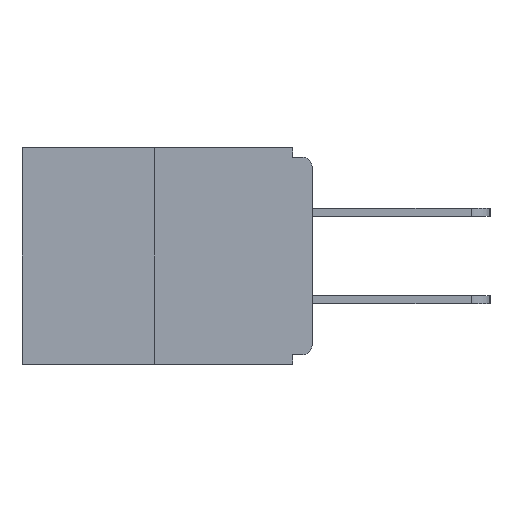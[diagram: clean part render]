
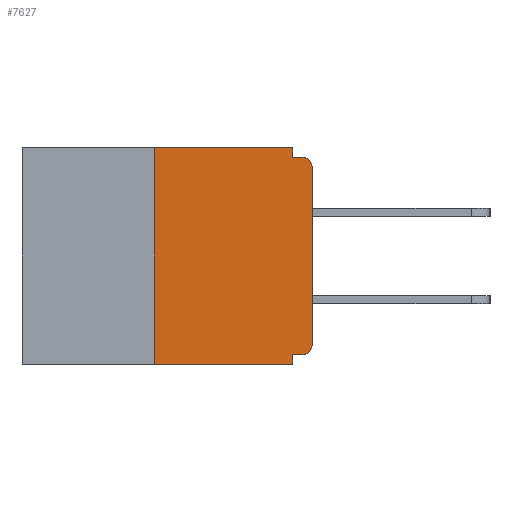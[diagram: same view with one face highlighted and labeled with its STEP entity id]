
A CAD part, left-side view. The second image highlights one B-rep face of the part: STEP entity #7627.
In plain terms, the highlighted planar face has unit normal (-1, 0, 0).
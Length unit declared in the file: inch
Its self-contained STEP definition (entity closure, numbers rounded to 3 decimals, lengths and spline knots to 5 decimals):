
#273 = ORIENTED_EDGE ( 'NONE', *, *, #18826, .F. ) ;
#470 = EDGE_LOOP ( 'NONE', ( #4976, #16208, #1547, #25998, #273, #16233, #20205, #10262, #1026, #14381 ) ) ;
#870 = VECTOR ( 'NONE', #19834, 39.37008 ) ;
#945 = DIRECTION ( 'NONE',  ( 1., 0., 0. ) ) ;
#1026 = ORIENTED_EDGE ( 'NONE', *, *, #16231, .F. ) ;
#1203 = DIRECTION ( 'NONE',  ( 0., 0., -1. ) ) ;
#1547 = ORIENTED_EDGE ( 'NONE', *, *, #17357, .T. ) ;
#2032 = VECTOR ( 'NONE', #5694, 39.37008 ) ;
#2045 = DIRECTION ( 'NONE',  ( 0., 0., 1. ) ) ;
#2410 = CARTESIAN_POINT ( 'NONE',  ( 0., 0.015, -0.313 ) ) ;
#3514 = DIRECTION ( 'NONE',  ( 0., -1., 0. ) ) ;
#3587 = LINE ( 'NONE', #8231, #18515 ) ;
#4628 = DIRECTION ( 'NONE',  ( -1., 0., 0. ) ) ;
#4914 = EDGE_CURVE ( 'NONE', #7676, #7644, #20408, .T. ) ;
#4976 = ORIENTED_EDGE ( 'NONE', *, *, #7115, .F. ) ;
#5045 = CARTESIAN_POINT ( 'NONE',  ( 0., 0.031, -0.015 ) ) ;
#5095 = EDGE_CURVE ( 'NONE', #22846, #19118, #3587, .T. ) ;
#5694 = DIRECTION ( 'NONE',  ( 0., -1., 0. ) ) ;
#6018 = CARTESIAN_POINT ( 'NONE',  ( 0., 0.031, 0. ) ) ;
#6121 = AXIS2_PLACEMENT_3D ( 'NONE', #2410, #4628, #24549 ) ;
#6451 = DIRECTION ( 'NONE',  ( -1., 0., 0. ) ) ;
#7105 = PLANE ( 'NONE',  #16457 ) ;
#7115 = EDGE_CURVE ( 'NONE', #15376, #7676, #24294, .T. ) ;
#7213 = CIRCLE ( 'NONE', #6121, 0.015 ) ;
#7627 = ADVANCED_FACE ( 'NONE', ( #17878 ), #7105, .F. ) ;
#7644 = VERTEX_POINT ( 'NONE', #5045 ) ;
#7676 = VERTEX_POINT ( 'NONE', #6018 ) ;
#7841 = CARTESIAN_POINT ( 'NONE',  ( 0., 0.46, 0. ) ) ;
#8231 = CARTESIAN_POINT ( 'NONE',  ( 0., 0., 0. ) ) ;
#8272 = CARTESIAN_POINT ( 'NONE',  ( 0., 0.015, -0.328 ) ) ;
#8774 = VERTEX_POINT ( 'NONE', #12982 ) ;
#8890 = LINE ( 'NONE', #25991, #870 ) ;
#8974 = CARTESIAN_POINT ( 'NONE',  ( 0., 0.015, -0.015 ) ) ;
#9414 = LINE ( 'NONE', #15908, #13529 ) ;
#9775 = DIRECTION ( 'NONE',  ( 0., 0., 1. ) ) ;
#10262 = ORIENTED_EDGE ( 'NONE', *, *, #13984, .T. ) ;
#11109 = CARTESIAN_POINT ( 'NONE',  ( 0., 0.46, 0. ) ) ;
#11891 = VERTEX_POINT ( 'NONE', #17225 ) ;
#12394 = AXIS2_PLACEMENT_3D ( 'NONE', #14437, #6451, #20337 ) ;
#12460 = CARTESIAN_POINT ( 'NONE',  ( 0., 0.25, 0. ) ) ;
#12982 = CARTESIAN_POINT ( 'NONE',  ( 0., 0.031, -0.328 ) ) ;
#13123 = CIRCLE ( 'NONE', #12394, 0.015 ) ;
#13529 = VECTOR ( 'NONE', #9775, 39.37008 ) ;
#13752 = VERTEX_POINT ( 'NONE', #8974 ) ;
#13984 = EDGE_CURVE ( 'NONE', #19118, #13752, #13123, .T. ) ;
#14179 = DIRECTION ( 'NONE',  ( 0., 0., -1. ) ) ;
#14381 = ORIENTED_EDGE ( 'NONE', *, *, #4914, .F. ) ;
#14437 = CARTESIAN_POINT ( 'NONE',  ( 0., 0.015, -0.03 ) ) ;
#15220 = VECTOR ( 'NONE', #20674, 39.37008 ) ;
#15376 = VERTEX_POINT ( 'NONE', #12460 ) ;
#15908 = CARTESIAN_POINT ( 'NONE',  ( 0., 0.25, 0. ) ) ;
#16152 = CARTESIAN_POINT ( 'NONE',  ( 0., 0.031, 0. ) ) ;
#16208 = ORIENTED_EDGE ( 'NONE', *, *, #24784, .F. ) ;
#16231 = EDGE_CURVE ( 'NONE', #7644, #13752, #20591, .T. ) ;
#16233 = ORIENTED_EDGE ( 'NONE', *, *, #24328, .T. ) ;
#16457 = AXIS2_PLACEMENT_3D ( 'NONE', #11109, #945, #1203 ) ;
#16479 = CARTESIAN_POINT ( 'NONE',  ( 0., 0.031, -0.343 ) ) ;
#16596 = LINE ( 'NONE', #16479, #21335 ) ;
#16727 = CARTESIAN_POINT ( 'NONE',  ( 0., 0., -0.313 ) ) ;
#17034 = VECTOR ( 'NONE', #3514, 39.37008 ) ;
#17225 = CARTESIAN_POINT ( 'NONE',  ( 0., 0.031, -0.343 ) ) ;
#17357 = EDGE_CURVE ( 'NONE', #17776, #11891, #17661, .T. ) ;
#17544 = CARTESIAN_POINT ( 'NONE',  ( 0., 0.46, -0.343 ) ) ;
#17566 = VECTOR ( 'NONE', #20380, 39.37008 ) ;
#17661 = LINE ( 'NONE', #17544, #17034 ) ;
#17776 = VERTEX_POINT ( 'NONE', #20984 ) ;
#17878 = FACE_OUTER_BOUND ( 'NONE', #470, .T. ) ;
#18515 = VECTOR ( 'NONE', #2045, 39.37008 ) ;
#18826 = EDGE_CURVE ( 'NONE', #25404, #8774, #8890, .T. ) ;
#18876 = CARTESIAN_POINT ( 'NONE',  ( 0., 0., -0.015 ) ) ;
#19118 = VERTEX_POINT ( 'NONE', #24388 ) ;
#19834 = DIRECTION ( 'NONE',  ( 0., 1., 0. ) ) ;
#20205 = ORIENTED_EDGE ( 'NONE', *, *, #5095, .T. ) ;
#20337 = DIRECTION ( 'NONE',  ( 0., 0., -1. ) ) ;
#20380 = DIRECTION ( 'NONE',  ( 0., 0., -1. ) ) ;
#20408 = LINE ( 'NONE', #16152, #17566 ) ;
#20591 = LINE ( 'NONE', #18876, #15220 ) ;
#20674 = DIRECTION ( 'NONE',  ( 0., -1., 0. ) ) ;
#20984 = CARTESIAN_POINT ( 'NONE',  ( 0., 0.25, -0.343 ) ) ;
#21335 = VECTOR ( 'NONE', #14179, 39.37008 ) ;
#21636 = EDGE_CURVE ( 'NONE', #8774, #11891, #16596, .T. ) ;
#22846 = VERTEX_POINT ( 'NONE', #16727 ) ;
#24294 = LINE ( 'NONE', #7841, #2032 ) ;
#24328 = EDGE_CURVE ( 'NONE', #25404, #22846, #7213, .T. ) ;
#24388 = CARTESIAN_POINT ( 'NONE',  ( 0., 0., -0.03 ) ) ;
#24549 = DIRECTION ( 'NONE',  ( 0., 0., -1. ) ) ;
#24784 = EDGE_CURVE ( 'NONE', #17776, #15376, #9414, .T. ) ;
#25404 = VERTEX_POINT ( 'NONE', #8272 ) ;
#25991 = CARTESIAN_POINT ( 'NONE',  ( 0., 0., -0.328 ) ) ;
#25998 = ORIENTED_EDGE ( 'NONE', *, *, #21636, .F. ) ;
